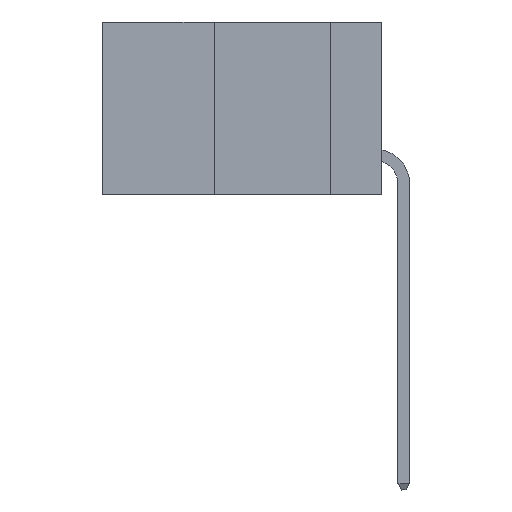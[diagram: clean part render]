
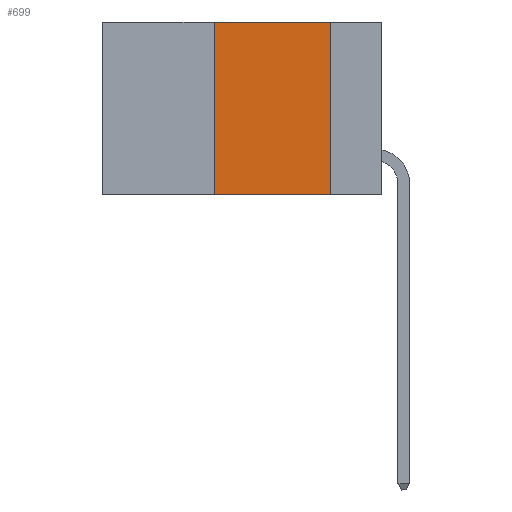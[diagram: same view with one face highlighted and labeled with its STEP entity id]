
A CAD part, left-side view. The second image highlights one B-rep face of the part: STEP entity #699.
In plain terms, the highlighted planar face has unit normal (-1, 0, 0).
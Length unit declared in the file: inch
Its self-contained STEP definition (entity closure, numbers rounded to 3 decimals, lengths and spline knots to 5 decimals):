
#683 = DIRECTION ( 'NONE',  ( 1., 0., 0. ) ) ;
#699 = ADVANCED_FACE ( 'NONE', ( #5606 ), #22952, .F. ) ;
#2422 = CARTESIAN_POINT ( 'NONE',  ( 0., 0.36, 0. ) ) ;
#2652 = DIRECTION ( 'NONE',  ( 0., 0., -1. ) ) ;
#2788 = VERTEX_POINT ( 'NONE', #19967 ) ;
#3537 = CARTESIAN_POINT ( 'NONE',  ( 0., 0.11, -0.37 ) ) ;
#3842 = LINE ( 'NONE', #23210, #12953 ) ;
#4911 = ORIENTED_EDGE ( 'NONE', *, *, #18034, .F. ) ;
#5606 = FACE_OUTER_BOUND ( 'NONE', #11798, .T. ) ;
#6363 = VECTOR ( 'NONE', #16677, 39.37008 ) ;
#7104 = CARTESIAN_POINT ( 'NONE',  ( 0., 0.36, 0. ) ) ;
#7588 = AXIS2_PLACEMENT_3D ( 'NONE', #8747, #683, #2652 ) ;
#7939 = LINE ( 'NONE', #18855, #6363 ) ;
#8268 = VECTOR ( 'NONE', #24492, 39.37008 ) ;
#8451 = CARTESIAN_POINT ( 'NONE',  ( 0., 0.6, -0.37 ) ) ;
#8747 = CARTESIAN_POINT ( 'NONE',  ( 0., 0.6, 0. ) ) ;
#11297 = ORIENTED_EDGE ( 'NONE', *, *, #14365, .F. ) ;
#11685 = ORIENTED_EDGE ( 'NONE', *, *, #25386, .F. ) ;
#11798 = EDGE_LOOP ( 'NONE', ( #4911, #11685, #11297, #23807 ) ) ;
#12229 = LINE ( 'NONE', #7104, #25559 ) ;
#12363 = CARTESIAN_POINT ( 'NONE',  ( 0., 0.11, 0. ) ) ;
#12790 = VERTEX_POINT ( 'NONE', #3537 ) ;
#12953 = VECTOR ( 'NONE', #23029, 39.37008 ) ;
#14365 = EDGE_CURVE ( 'NONE', #2788, #24134, #12229, .T. ) ;
#16221 = VERTEX_POINT ( 'NONE', #12363 ) ;
#16677 = DIRECTION ( 'NONE',  ( 0., 0., -1. ) ) ;
#17433 = LINE ( 'NONE', #8451, #8268 ) ;
#17811 = EDGE_CURVE ( 'NONE', #2788, #12790, #17433, .T. ) ;
#18034 = EDGE_CURVE ( 'NONE', #16221, #12790, #7939, .T. ) ;
#18855 = CARTESIAN_POINT ( 'NONE',  ( 0., 0.11, 0. ) ) ;
#19088 = DIRECTION ( 'NONE',  ( 0., 0., 1. ) ) ;
#19967 = CARTESIAN_POINT ( 'NONE',  ( 0., 0.36, -0.37 ) ) ;
#22952 = PLANE ( 'NONE',  #7588 ) ;
#23029 = DIRECTION ( 'NONE',  ( 0., -1., 0. ) ) ;
#23210 = CARTESIAN_POINT ( 'NONE',  ( 0., 0.6, 0. ) ) ;
#23807 = ORIENTED_EDGE ( 'NONE', *, *, #17811, .T. ) ;
#24134 = VERTEX_POINT ( 'NONE', #2422 ) ;
#24492 = DIRECTION ( 'NONE',  ( 0., -1., 0. ) ) ;
#25386 = EDGE_CURVE ( 'NONE', #24134, #16221, #3842, .T. ) ;
#25559 = VECTOR ( 'NONE', #19088, 39.37008 ) ;
